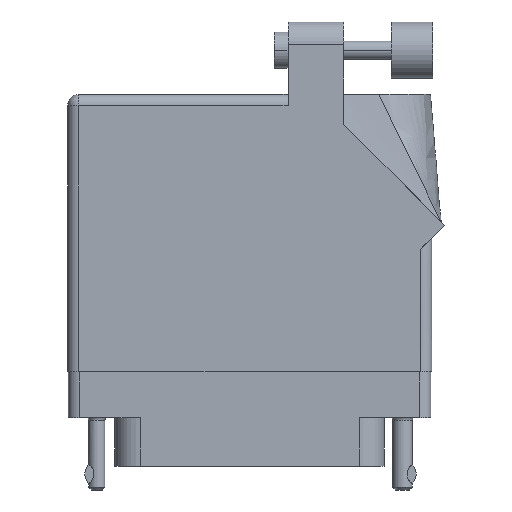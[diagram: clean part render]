
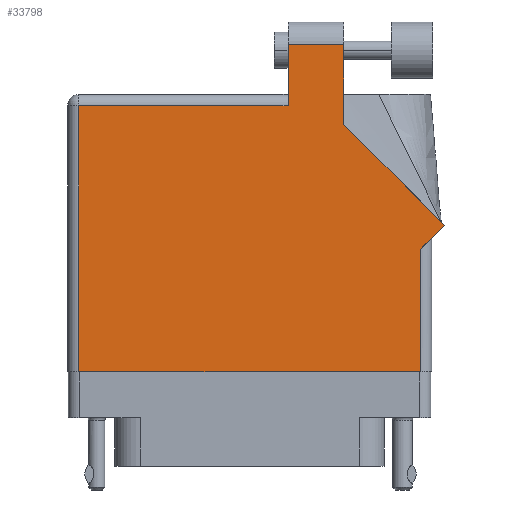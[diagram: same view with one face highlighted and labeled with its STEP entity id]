
A CAD part, front view. The second image highlights one B-rep face of the part: STEP entity #33798.
In plain terms, the highlighted face is planar.
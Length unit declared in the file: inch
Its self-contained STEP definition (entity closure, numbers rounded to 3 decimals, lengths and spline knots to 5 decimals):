
#95 = DIRECTION ( 'NONE',  ( -1., 0., 0. ) ) ;
#281 = ORIENTED_EDGE ( 'NONE', *, *, #14030, .T. ) ;
#414 = CARTESIAN_POINT ( 'NONE',  ( 1.005, 0.637, 0.455 ) ) ;
#742 = VERTEX_POINT ( 'NONE', #25702 ) ;
#1244 = CARTESIAN_POINT ( 'NONE',  ( -0.943, 1.368, 0.455 ) ) ;
#1752 = CARTESIAN_POINT ( 'NONE',  ( 0.212, 1.705, 0.455 ) ) ;
#2670 = VECTOR ( 'NONE', #30424, 39.37008 ) ;
#3024 = LINE ( 'NONE', #22229, #4579 ) ;
#3567 = LINE ( 'NONE', #19282, #11553 ) ;
#3719 = EDGE_CURVE ( 'NONE', #31056, #18999, #39130, .T. ) ;
#4020 = CARTESIAN_POINT ( 'NONE',  ( 1.07571, 0.70771, 0.455 ) ) ;
#4579 = VECTOR ( 'NONE', #29265, 39.37008 ) ;
#4629 = DIRECTION ( 'NONE',  ( 0.707, 0.707, 0. ) ) ;
#4732 = LINE ( 'NONE', #5254, #9842 ) ;
#5254 = CARTESIAN_POINT ( 'NONE',  ( -0.943, -0.1, 0.455 ) ) ;
#6752 = ORIENTED_EDGE ( 'NONE', *, *, #42422, .T. ) ;
#7225 = CARTESIAN_POINT ( 'NONE',  ( -1.005, 1.43, 0.455 ) ) ;
#8726 = DIRECTION ( 'NONE',  ( 0., -1., 0. ) ) ;
#9842 = VECTOR ( 'NONE', #8726, 39.37008 ) ;
#9997 = VECTOR ( 'NONE', #23681, 39.37008 ) ;
#10254 = ORIENTED_EDGE ( 'NONE', *, *, #31389, .T. ) ;
#10467 = VECTOR ( 'NONE', #4629, 39.37008 ) ;
#11379 = CARTESIAN_POINT ( 'NONE',  ( 0.212, 1.368, 0.455 ) ) ;
#11537 = CARTESIAN_POINT ( 'NONE',  ( -1.005, 1.368, 0.455 ) ) ;
#11553 = VECTOR ( 'NONE', #14789, 39.37008 ) ;
#13337 = AXIS2_PLACEMENT_3D ( 'NONE', #7225, #30690, #37921 ) ;
#13360 = CARTESIAN_POINT ( 'NONE',  ( -0.943, -0.1, 0.455 ) ) ;
#14030 = EDGE_CURVE ( 'NONE', #18999, #30423, #19301, .T. ) ;
#14789 = DIRECTION ( 'NONE',  ( 1., 0., 0. ) ) ;
#14896 = VERTEX_POINT ( 'NONE', #18180 ) ;
#15174 = CARTESIAN_POINT ( 'NONE',  ( 0.943, 0.637, 0.455 ) ) ;
#15974 = VERTEX_POINT ( 'NONE', #4020 ) ;
#18180 = CARTESIAN_POINT ( 'NONE',  ( 0.943, 0.575, 0.455 ) ) ;
#18805 = CARTESIAN_POINT ( 'NONE',  ( 0.212, 1.43, 0.455 ) ) ;
#18818 = CARTESIAN_POINT ( 'NONE',  ( 0.519, 1.26442, 0.455 ) ) ;
#18999 = VERTEX_POINT ( 'NONE', #1752 ) ;
#19282 = CARTESIAN_POINT ( 'NONE',  ( -1.005, -0.1, 0.455 ) ) ;
#19301 = LINE ( 'NONE', #18805, #44332 ) ;
#19928 = CARTESIAN_POINT ( 'NONE',  ( 0.212, 1.705, 0.455 ) ) ;
#22229 = CARTESIAN_POINT ( 'NONE',  ( 1.07571, 0.70771, 0.455 ) ) ;
#23526 = ORIENTED_EDGE ( 'NONE', *, *, #39016, .T. ) ;
#23681 = DIRECTION ( 'NONE',  ( -1., 0., 0. ) ) ;
#24321 = CARTESIAN_POINT ( 'NONE',  ( 0.519, 1.705, 0.455 ) ) ;
#25555 = EDGE_CURVE ( 'NONE', #30423, #30133, #27551, .T. ) ;
#25702 = CARTESIAN_POINT ( 'NONE',  ( 0.519, 1.26442, 0.455 ) ) ;
#26950 = FACE_OUTER_BOUND ( 'NONE', #31216, .T. ) ;
#27043 = DIRECTION ( 'NONE',  ( 0., -1., 0. ) ) ;
#27551 = LINE ( 'NONE', #11537, #38503 ) ;
#29127 = EDGE_CURVE ( 'NONE', #34073, #14896, #29950, .T. ) ;
#29226 = ORIENTED_EDGE ( 'NONE', *, *, #3719, .T. ) ;
#29265 = DIRECTION ( 'NONE',  ( -0.707, 0.707, 0. ) ) ;
#29950 = LINE ( 'NONE', #15174, #2670 ) ;
#30064 = EDGE_CURVE ( 'NONE', #742, #31056, #33320, .T. ) ;
#30133 = VERTEX_POINT ( 'NONE', #1244 ) ;
#30423 = VERTEX_POINT ( 'NONE', #11379 ) ;
#30424 = DIRECTION ( 'NONE',  ( 0., 1., 0. ) ) ;
#30690 = DIRECTION ( 'NONE',  ( 0., 0., -1. ) ) ;
#30754 = VERTEX_POINT ( 'NONE', #13360 ) ;
#31056 = VERTEX_POINT ( 'NONE', #24321 ) ;
#31216 = EDGE_LOOP ( 'NONE', ( #32759, #29226, #281, #35180, #42267, #10254, #47233, #23526, #6752 ) ) ;
#31389 = EDGE_CURVE ( 'NONE', #30754, #34073, #3567, .T. ) ;
#32759 = ORIENTED_EDGE ( 'NONE', *, *, #30064, .T. ) ;
#33320 = LINE ( 'NONE', #18818, #43412 ) ;
#33798 = ADVANCED_FACE ( 'NONE', ( #26950 ), #48910, .F. ) ;
#34047 = DIRECTION ( 'NONE',  ( 0., 1., 0. ) ) ;
#34073 = VERTEX_POINT ( 'NONE', #48316 ) ;
#35180 = ORIENTED_EDGE ( 'NONE', *, *, #25555, .T. ) ;
#37921 = DIRECTION ( 'NONE',  ( -1., 0., 0. ) ) ;
#38503 = VECTOR ( 'NONE', #95, 39.37008 ) ;
#38807 = LINE ( 'NONE', #414, #10467 ) ;
#39016 = EDGE_CURVE ( 'NONE', #14896, #15974, #38807, .T. ) ;
#39130 = LINE ( 'NONE', #19928, #9997 ) ;
#41137 = EDGE_CURVE ( 'NONE', #30133, #30754, #4732, .T. ) ;
#42267 = ORIENTED_EDGE ( 'NONE', *, *, #41137, .T. ) ;
#42422 = EDGE_CURVE ( 'NONE', #15974, #742, #3024, .T. ) ;
#43412 = VECTOR ( 'NONE', #34047, 39.37008 ) ;
#44332 = VECTOR ( 'NONE', #27043, 39.37008 ) ;
#47233 = ORIENTED_EDGE ( 'NONE', *, *, #29127, .T. ) ;
#48316 = CARTESIAN_POINT ( 'NONE',  ( 0.943, -0.1, 0.455 ) ) ;
#48910 = PLANE ( 'NONE',  #13337 ) ;
